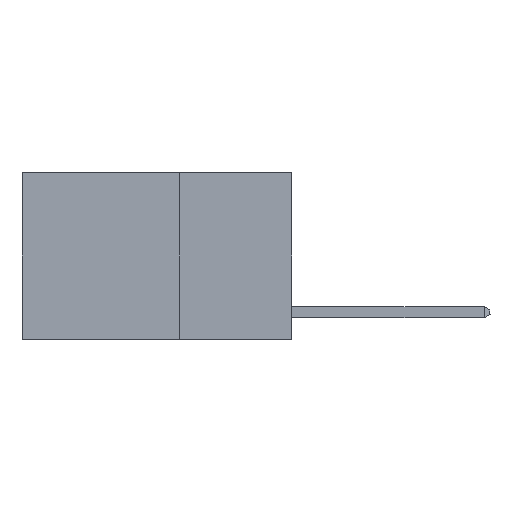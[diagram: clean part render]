
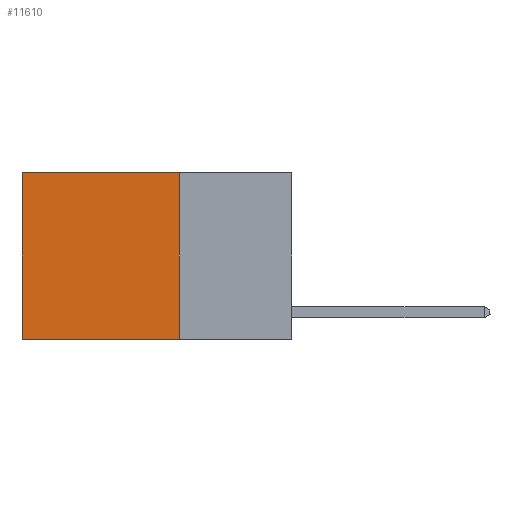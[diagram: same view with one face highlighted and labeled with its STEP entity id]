
A CAD part, left-side view. The second image highlights one B-rep face of the part: STEP entity #11610.
In plain terms, the highlighted planar face has unit normal (-1, 0, 0).
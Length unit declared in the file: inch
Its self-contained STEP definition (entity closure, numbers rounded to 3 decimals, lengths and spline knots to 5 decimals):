
#1283 = EDGE_CURVE ( 'NONE', #13112, #6654, #3713, .T. ) ;
#1712 = CARTESIAN_POINT ( 'NONE',  ( 0.2625, 0.25, 0. ) ) ;
#1903 = DIRECTION ( 'NONE',  ( 0., 0., -1. ) ) ;
#2492 = CARTESIAN_POINT ( 'NONE',  ( 0.2625, 0.25, 0. ) ) ;
#3192 = EDGE_CURVE ( 'NONE', #8337, #16844, #3854, .T. ) ;
#3713 = LINE ( 'NONE', #11840, #11275 ) ;
#3854 = LINE ( 'NONE', #1712, #14721 ) ;
#4156 = CARTESIAN_POINT ( 'NONE',  ( 0.2625, 0.25, -0.37 ) ) ;
#4559 = DIRECTION ( 'NONE',  ( 0., 0., -1. ) ) ;
#4883 = ORIENTED_EDGE ( 'NONE', *, *, #1283, .T. ) ;
#5529 = EDGE_CURVE ( 'NONE', #8337, #13112, #12394, .T. ) ;
#6654 = VERTEX_POINT ( 'NONE', #10611 ) ;
#6750 = PLANE ( 'NONE',  #7803 ) ;
#7803 = AXIS2_PLACEMENT_3D ( 'NONE', #2492, #16646, #8206 ) ;
#8206 = DIRECTION ( 'NONE',  ( 0., 0., -1. ) ) ;
#8216 = EDGE_CURVE ( 'NONE', #16844, #6654, #17959, .T. ) ;
#8337 = VERTEX_POINT ( 'NONE', #15713 ) ;
#8399 = DIRECTION ( 'NONE',  ( 0., 1., 0. ) ) ;
#8598 = VECTOR ( 'NONE', #11271, 39.37008 ) ;
#10611 = CARTESIAN_POINT ( 'NONE',  ( 0.2625, 0.6, -0.37 ) ) ;
#11071 = CARTESIAN_POINT ( 'NONE',  ( 0.2625, 0.6, 0. ) ) ;
#11271 = DIRECTION ( 'NONE',  ( 0., 1., 0. ) ) ;
#11275 = VECTOR ( 'NONE', #1903, 39.37008 ) ;
#11534 = FACE_OUTER_BOUND ( 'NONE', #16464, .T. ) ;
#11610 = ADVANCED_FACE ( 'NONE', ( #11534 ), #6750, .F. ) ;
#11834 = ORIENTED_EDGE ( 'NONE', *, *, #5529, .T. ) ;
#11840 = CARTESIAN_POINT ( 'NONE',  ( 0.2625, 0.6, 0. ) ) ;
#12394 = LINE ( 'NONE', #18251, #8598 ) ;
#13112 = VERTEX_POINT ( 'NONE', #11071 ) ;
#13521 = CARTESIAN_POINT ( 'NONE',  ( 0.2625, 0.25, -0.37 ) ) ;
#13554 = ORIENTED_EDGE ( 'NONE', *, *, #8216, .F. ) ;
#13819 = VECTOR ( 'NONE', #8399, 39.37008 ) ;
#14721 = VECTOR ( 'NONE', #4559, 39.37008 ) ;
#15713 = CARTESIAN_POINT ( 'NONE',  ( 0.2625, 0.25, 0. ) ) ;
#16464 = EDGE_LOOP ( 'NONE', ( #4883, #13554, #17005, #11834 ) ) ;
#16646 = DIRECTION ( 'NONE',  ( 1., 0., 0. ) ) ;
#16844 = VERTEX_POINT ( 'NONE', #13521 ) ;
#17005 = ORIENTED_EDGE ( 'NONE', *, *, #3192, .F. ) ;
#17959 = LINE ( 'NONE', #4156, #13819 ) ;
#18251 = CARTESIAN_POINT ( 'NONE',  ( 0.2625, 0.25, 0. ) ) ;
